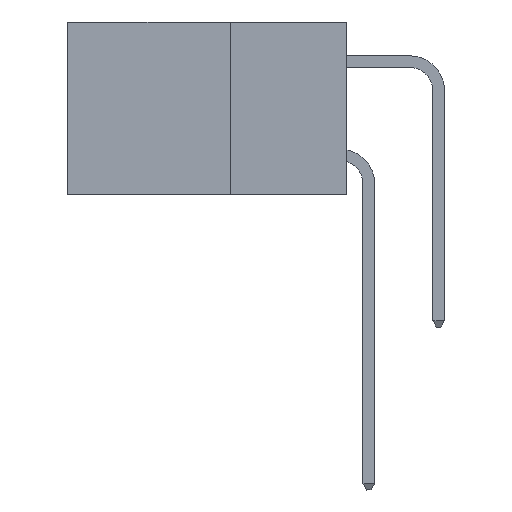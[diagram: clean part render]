
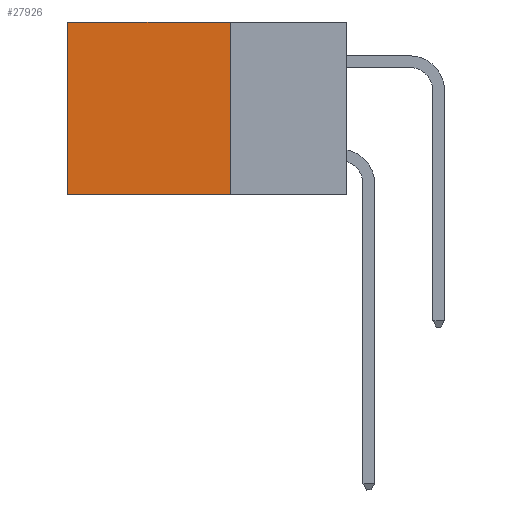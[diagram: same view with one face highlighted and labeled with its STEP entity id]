
A CAD part, left-side view. The second image highlights one B-rep face of the part: STEP entity #27926.
In plain terms, the highlighted planar face has unit normal (-1, 0, 0).
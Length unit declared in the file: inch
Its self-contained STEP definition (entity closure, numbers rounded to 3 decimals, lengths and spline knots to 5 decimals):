
#477 = CARTESIAN_POINT ( 'NONE',  ( 0.2875, 0.6, 0. ) ) ;
#716 = DIRECTION ( 'NONE',  ( 0., 1., 0. ) ) ;
#1337 = DIRECTION ( 'NONE',  ( 0., 0., -1. ) ) ;
#3284 = LINE ( 'NONE', #38451, #19505 ) ;
#5034 = CARTESIAN_POINT ( 'NONE',  ( 0.2875, 0.6, 0. ) ) ;
#5868 = CARTESIAN_POINT ( 'NONE',  ( 0.2875, 0.25, 0. ) ) ;
#6270 = EDGE_CURVE ( 'NONE', #37922, #25001, #18977, .T. ) ;
#8212 = ORIENTED_EDGE ( 'NONE', *, *, #40445, .F. ) ;
#9341 = AXIS2_PLACEMENT_3D ( 'NONE', #5868, #9366, #35431 ) ;
#9366 = DIRECTION ( 'NONE',  ( 1., 0., 0. ) ) ;
#9584 = VECTOR ( 'NONE', #1337, 39.37008 ) ;
#11839 = LINE ( 'NONE', #27162, #23823 ) ;
#14324 = ORIENTED_EDGE ( 'NONE', *, *, #6270, .T. ) ;
#15812 = FACE_OUTER_BOUND ( 'NONE', #15926, .T. ) ;
#15926 = EDGE_LOOP ( 'NONE', ( #14324, #32133, #8212, #39570 ) ) ;
#18639 = CARTESIAN_POINT ( 'NONE',  ( 0.2875, 0.25, -0.37 ) ) ;
#18977 = LINE ( 'NONE', #477, #9584 ) ;
#19505 = VECTOR ( 'NONE', #35554, 39.37008 ) ;
#22638 = EDGE_CURVE ( 'NONE', #23134, #25001, #3284, .T. ) ;
#22994 = LINE ( 'NONE', #25709, #30268 ) ;
#23134 = VERTEX_POINT ( 'NONE', #18639 ) ;
#23823 = VECTOR ( 'NONE', #716, 39.37008 ) ;
#25001 = VERTEX_POINT ( 'NONE', #25242 ) ;
#25242 = CARTESIAN_POINT ( 'NONE',  ( 0.2875, 0.6, -0.37 ) ) ;
#25709 = CARTESIAN_POINT ( 'NONE',  ( 0.2875, 0.25, 0. ) ) ;
#25913 = PLANE ( 'NONE',  #9341 ) ;
#26558 = CARTESIAN_POINT ( 'NONE',  ( 0.2875, 0.25, 0. ) ) ;
#27162 = CARTESIAN_POINT ( 'NONE',  ( 0.2875, 0.25, 0. ) ) ;
#27926 = ADVANCED_FACE ( 'NONE', ( #15812 ), #25913, .F. ) ;
#30268 = VECTOR ( 'NONE', #35923, 39.37008 ) ;
#31466 = VERTEX_POINT ( 'NONE', #26558 ) ;
#32133 = ORIENTED_EDGE ( 'NONE', *, *, #22638, .F. ) ;
#35431 = DIRECTION ( 'NONE',  ( 0., 0., -1. ) ) ;
#35554 = DIRECTION ( 'NONE',  ( 0., 1., 0. ) ) ;
#35923 = DIRECTION ( 'NONE',  ( 0., 0., -1. ) ) ;
#37922 = VERTEX_POINT ( 'NONE', #5034 ) ;
#38451 = CARTESIAN_POINT ( 'NONE',  ( 0.2875, 0.25, -0.37 ) ) ;
#38981 = EDGE_CURVE ( 'NONE', #31466, #37922, #11839, .T. ) ;
#39570 = ORIENTED_EDGE ( 'NONE', *, *, #38981, .T. ) ;
#40445 = EDGE_CURVE ( 'NONE', #31466, #23134, #22994, .T. ) ;
